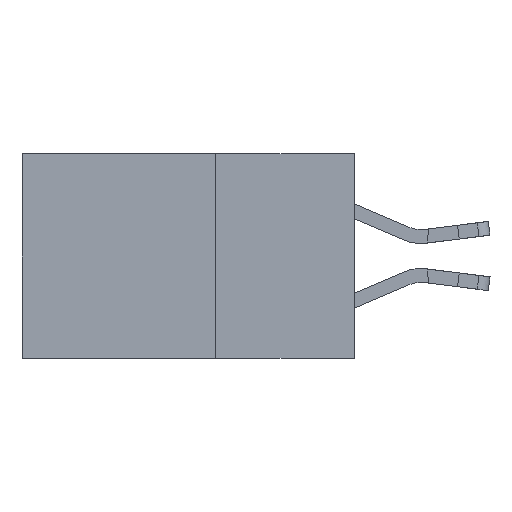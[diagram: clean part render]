
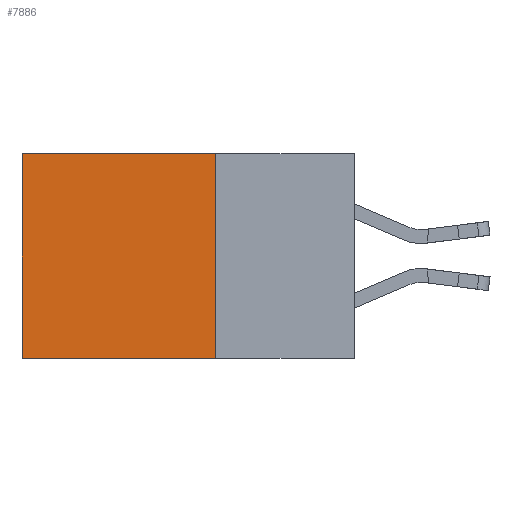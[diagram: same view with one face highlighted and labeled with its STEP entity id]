
A CAD part, left-side view. The second image highlights one B-rep face of the part: STEP entity #7886.
In plain terms, the highlighted planar face has unit normal (-1, 0, 0).
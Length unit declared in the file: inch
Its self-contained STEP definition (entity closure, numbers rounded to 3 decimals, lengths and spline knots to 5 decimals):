
#1062 = VECTOR ( 'NONE', #4879, 39.37008 ) ;
#1113 = CARTESIAN_POINT ( 'NONE',  ( 0.2615, 0.25, -0.37 ) ) ;
#1744 = EDGE_CURVE ( 'NONE', #4686, #4286, #4414, .T. ) ;
#3361 = DIRECTION ( 'NONE',  ( 0., 1., 0. ) ) ;
#3816 = ORIENTED_EDGE ( 'NONE', *, *, #1744, .T. ) ;
#4286 = VERTEX_POINT ( 'NONE', #10367 ) ;
#4414 = LINE ( 'NONE', #10179, #14487 ) ;
#4686 = VERTEX_POINT ( 'NONE', #7149 ) ;
#4879 = DIRECTION ( 'NONE',  ( 0., 0., -1. ) ) ;
#4936 = EDGE_CURVE ( 'NONE', #4286, #16325, #12144, .T. ) ;
#5209 = ORIENTED_EDGE ( 'NONE', *, *, #4936, .T. ) ;
#5251 = CARTESIAN_POINT ( 'NONE',  ( 0.2615, 0.6, -0.37 ) ) ;
#5726 = VECTOR ( 'NONE', #3361, 39.37008 ) ;
#7149 = CARTESIAN_POINT ( 'NONE',  ( 0.2615, 0.25, 0. ) ) ;
#7886 = ADVANCED_FACE ( 'NONE', ( #10512 ), #9943, .F. ) ;
#8523 = EDGE_CURVE ( 'NONE', #14601, #16325, #13054, .T. ) ;
#8805 = ORIENTED_EDGE ( 'NONE', *, *, #16281, .F. ) ;
#9570 = ORIENTED_EDGE ( 'NONE', *, *, #8523, .F. ) ;
#9828 = DIRECTION ( 'NONE',  ( 0., 1., 0. ) ) ;
#9875 = DIRECTION ( 'NONE',  ( 0., 0., -1. ) ) ;
#9894 = DIRECTION ( 'NONE',  ( 1., 0., 0. ) ) ;
#9915 = CARTESIAN_POINT ( 'NONE',  ( 0.2615, 0.25, -0.37 ) ) ;
#9943 = PLANE ( 'NONE',  #17752 ) ;
#10179 = CARTESIAN_POINT ( 'NONE',  ( 0.2615, 0.25, 0. ) ) ;
#10188 = CARTESIAN_POINT ( 'NONE',  ( 0.2615, 0.25, -0.37 ) ) ;
#10367 = CARTESIAN_POINT ( 'NONE',  ( 0.2615, 0.6, 0. ) ) ;
#10512 = FACE_OUTER_BOUND ( 'NONE', #15619, .T. ) ;
#11117 = LINE ( 'NONE', #13709, #11551 ) ;
#11551 = VECTOR ( 'NONE', #16399, 39.37008 ) ;
#12144 = LINE ( 'NONE', #5251, #1062 ) ;
#13054 = LINE ( 'NONE', #10188, #5726 ) ;
#13709 = CARTESIAN_POINT ( 'NONE',  ( 0.2615, 0.25, -0.37 ) ) ;
#13771 = CARTESIAN_POINT ( 'NONE',  ( 0.2615, 0.6, -0.37 ) ) ;
#14487 = VECTOR ( 'NONE', #9828, 39.37008 ) ;
#14601 = VERTEX_POINT ( 'NONE', #1113 ) ;
#15619 = EDGE_LOOP ( 'NONE', ( #5209, #9570, #8805, #3816 ) ) ;
#16281 = EDGE_CURVE ( 'NONE', #4686, #14601, #11117, .T. ) ;
#16325 = VERTEX_POINT ( 'NONE', #13771 ) ;
#16399 = DIRECTION ( 'NONE',  ( 0., 0., -1. ) ) ;
#17752 = AXIS2_PLACEMENT_3D ( 'NONE', #9915, #9894, #9875 ) ;
